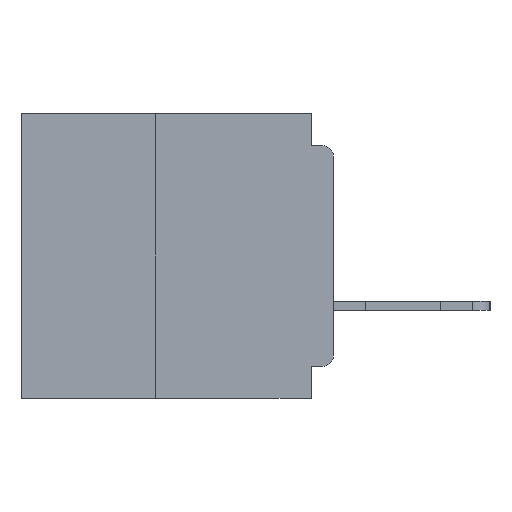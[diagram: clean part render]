
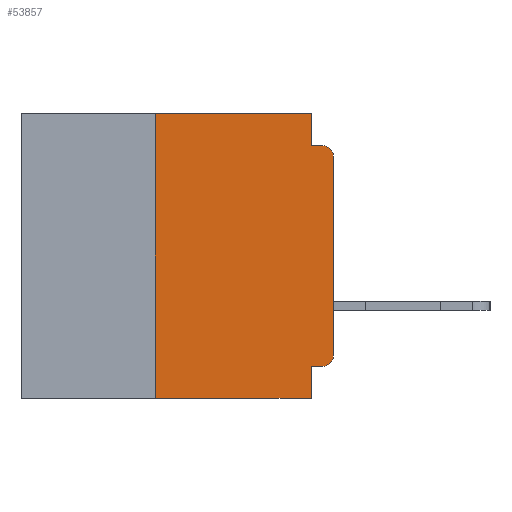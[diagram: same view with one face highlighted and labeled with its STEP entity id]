
A CAD part, left-side view. The second image highlights one B-rep face of the part: STEP entity #53857.
In plain terms, the highlighted planar face has unit normal (-1, 0, 0).
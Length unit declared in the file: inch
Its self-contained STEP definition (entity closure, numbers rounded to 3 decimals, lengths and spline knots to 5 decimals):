
#1843 = VERTEX_POINT ( 'NONE', #43382 ) ;
#1919 = CARTESIAN_POINT ( 'NONE',  ( 0., 0.015, -0.34 ) ) ;
#2332 = CARTESIAN_POINT ( 'NONE',  ( 0., 0., 0. ) ) ;
#2342 = VECTOR ( 'NONE', #44248, 39.37008 ) ;
#3039 = CARTESIAN_POINT ( 'NONE',  ( 0., 0.031, -0.355 ) ) ;
#3207 = VERTEX_POINT ( 'NONE', #31910 ) ;
#5234 = CARTESIAN_POINT ( 'NONE',  ( 0., 0.031, -0.4 ) ) ;
#6444 = DIRECTION ( 'NONE',  ( 0., 0., -1. ) ) ;
#6847 = CARTESIAN_POINT ( 'NONE',  ( 0., 0.437, 0. ) ) ;
#7057 = EDGE_CURVE ( 'NONE', #3207, #37009, #25709, .T. ) ;
#7059 = CIRCLE ( 'NONE', #26088, 0.015 ) ;
#8732 = ORIENTED_EDGE ( 'NONE', *, *, #30901, .F. ) ;
#8974 = ORIENTED_EDGE ( 'NONE', *, *, #56525, .T. ) ;
#9433 = LINE ( 'NONE', #2332, #56983 ) ;
#9463 = VECTOR ( 'NONE', #46419, 39.37008 ) ;
#9944 = EDGE_LOOP ( 'NONE', ( #19159, #8974, #57037, #37132, #21148, #27193, #51051, #32322, #8732, #10009 ) ) ;
#10009 = ORIENTED_EDGE ( 'NONE', *, *, #39627, .T. ) ;
#12185 = DIRECTION ( 'NONE',  ( 0., -1., 0. ) ) ;
#12377 = VECTOR ( 'NONE', #54005, 39.37008 ) ;
#12929 = CARTESIAN_POINT ( 'NONE',  ( 0., 0., -0.355 ) ) ;
#13280 = VERTEX_POINT ( 'NONE', #3039 ) ;
#13630 = VECTOR ( 'NONE', #54464, 39.37008 ) ;
#13930 = FACE_OUTER_BOUND ( 'NONE', #9944, .T. ) ;
#14853 = LINE ( 'NONE', #44167, #37283 ) ;
#17149 = LINE ( 'NONE', #5234, #38148 ) ;
#17250 = DIRECTION ( 'NONE',  ( -1., 0., 0. ) ) ;
#17799 = CIRCLE ( 'NONE', #28162, 0.015 ) ;
#19159 = ORIENTED_EDGE ( 'NONE', *, *, #20121, .T. ) ;
#20121 = EDGE_CURVE ( 'NONE', #32533, #32886, #9433, .T. ) ;
#20374 = PLANE ( 'NONE',  #42283 ) ;
#21148 = ORIENTED_EDGE ( 'NONE', *, *, #53397, .F. ) ;
#21217 = CARTESIAN_POINT ( 'NONE',  ( 0., 0.437, 0. ) ) ;
#22651 = CARTESIAN_POINT ( 'NONE',  ( 0., 0., -0.06 ) ) ;
#23209 = CARTESIAN_POINT ( 'NONE',  ( 0., 0.031, 0. ) ) ;
#23876 = EDGE_CURVE ( 'NONE', #13280, #1843, #17149, .T. ) ;
#24879 = DIRECTION ( 'NONE',  ( 1., 0., 0. ) ) ;
#25709 = LINE ( 'NONE', #27049, #12377 ) ;
#26088 = AXIS2_PLACEMENT_3D ( 'NONE', #1919, #33274, #6444 ) ;
#26982 = CARTESIAN_POINT ( 'NONE',  ( 0., 0.015, -0.045 ) ) ;
#27049 = CARTESIAN_POINT ( 'NONE',  ( 0., 0., -0.045 ) ) ;
#27193 = ORIENTED_EDGE ( 'NONE', *, *, #48265, .F. ) ;
#27777 = DIRECTION ( 'NONE',  ( 0., 0., -1. ) ) ;
#28162 = AXIS2_PLACEMENT_3D ( 'NONE', #44039, #17250, #48544 ) ;
#28953 = CARTESIAN_POINT ( 'NONE',  ( 0., 0., -0.34 ) ) ;
#29189 = DIRECTION ( 'NONE',  ( 0., 0., 1. ) ) ;
#30389 = CARTESIAN_POINT ( 'NONE',  ( 0., 0.015, -0.355 ) ) ;
#30901 = EDGE_CURVE ( 'NONE', #41384, #13280, #46578, .T. ) ;
#31910 = CARTESIAN_POINT ( 'NONE',  ( 0., 0.031, -0.045 ) ) ;
#31936 = VERTEX_POINT ( 'NONE', #56605 ) ;
#32322 = ORIENTED_EDGE ( 'NONE', *, *, #23876, .F. ) ;
#32533 = VERTEX_POINT ( 'NONE', #28953 ) ;
#32886 = VERTEX_POINT ( 'NONE', #22651 ) ;
#33274 = DIRECTION ( 'NONE',  ( -1., 0., 0. ) ) ;
#33296 = LINE ( 'NONE', #41924, #9463 ) ;
#37009 = VERTEX_POINT ( 'NONE', #26982 ) ;
#37132 = ORIENTED_EDGE ( 'NONE', *, *, #50736, .F. ) ;
#37283 = VECTOR ( 'NONE', #48666, 39.37008 ) ;
#37468 = LINE ( 'NONE', #23209, #13630 ) ;
#37817 = VECTOR ( 'NONE', #12185, 39.37008 ) ;
#38148 = VECTOR ( 'NONE', #27777, 39.37008 ) ;
#38202 = CARTESIAN_POINT ( 'NONE',  ( 0., 0.031, 0. ) ) ;
#39188 = VERTEX_POINT ( 'NONE', #38202 ) ;
#39627 = EDGE_CURVE ( 'NONE', #41384, #32533, #7059, .T. ) ;
#39688 = CARTESIAN_POINT ( 'NONE',  ( 0., 0.25, 0. ) ) ;
#41384 = VERTEX_POINT ( 'NONE', #30389 ) ;
#41924 = CARTESIAN_POINT ( 'NONE',  ( 0., 0.437, -0.4 ) ) ;
#42283 = AXIS2_PLACEMENT_3D ( 'NONE', #6847, #24879, #56103 ) ;
#43382 = CARTESIAN_POINT ( 'NONE',  ( 0., 0.031, -0.4 ) ) ;
#44039 = CARTESIAN_POINT ( 'NONE',  ( 0., 0.015, -0.06 ) ) ;
#44167 = CARTESIAN_POINT ( 'NONE',  ( 0., 0.25, -0.4 ) ) ;
#44248 = DIRECTION ( 'NONE',  ( 0., 1., 0. ) ) ;
#46419 = DIRECTION ( 'NONE',  ( 0., -1., 0. ) ) ;
#46578 = LINE ( 'NONE', #12929, #2342 ) ;
#47341 = EDGE_CURVE ( 'NONE', #31936, #1843, #33296, .T. ) ;
#48261 = VERTEX_POINT ( 'NONE', #39688 ) ;
#48265 = EDGE_CURVE ( 'NONE', #31936, #48261, #14853, .T. ) ;
#48544 = DIRECTION ( 'NONE',  ( 0., 0., -1. ) ) ;
#48666 = DIRECTION ( 'NONE',  ( 0., 0., 1. ) ) ;
#50736 = EDGE_CURVE ( 'NONE', #39188, #3207, #37468, .T. ) ;
#51051 = ORIENTED_EDGE ( 'NONE', *, *, #47341, .T. ) ;
#52468 = LINE ( 'NONE', #21217, #37817 ) ;
#53397 = EDGE_CURVE ( 'NONE', #48261, #39188, #52468, .T. ) ;
#53857 = ADVANCED_FACE ( 'NONE', ( #13930 ), #20374, .F. ) ;
#54005 = DIRECTION ( 'NONE',  ( 0., -1., 0. ) ) ;
#54464 = DIRECTION ( 'NONE',  ( 0., 0., -1. ) ) ;
#56103 = DIRECTION ( 'NONE',  ( 0., 0., -1. ) ) ;
#56525 = EDGE_CURVE ( 'NONE', #32886, #37009, #17799, .T. ) ;
#56605 = CARTESIAN_POINT ( 'NONE',  ( 0., 0.25, -0.4 ) ) ;
#56983 = VECTOR ( 'NONE', #29189, 39.37008 ) ;
#57037 = ORIENTED_EDGE ( 'NONE', *, *, #7057, .F. ) ;
